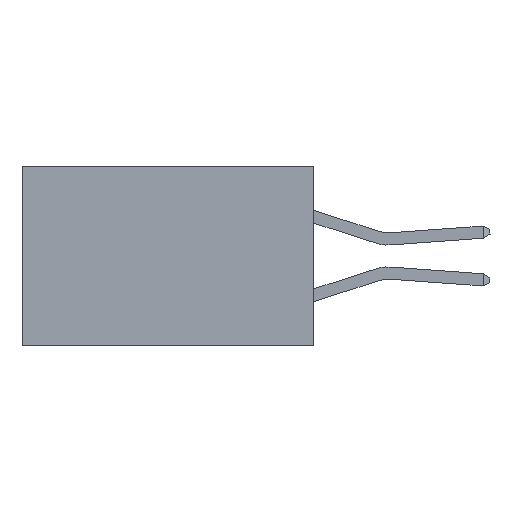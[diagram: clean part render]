
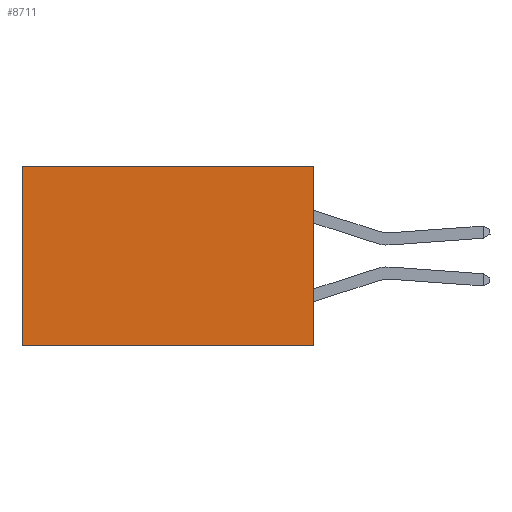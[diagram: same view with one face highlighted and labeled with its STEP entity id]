
A CAD part, left-side view. The second image highlights one B-rep face of the part: STEP entity #8711.
In plain terms, the highlighted planar face has unit normal (-1, 0, 0).
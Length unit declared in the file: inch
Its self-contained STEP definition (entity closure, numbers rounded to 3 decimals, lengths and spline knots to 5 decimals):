
#240 = LINE ( 'NONE', #2811, #2835 ) ;
#1067 = DIRECTION ( 'NONE',  ( 1., 0., 0. ) ) ;
#1459 = LINE ( 'NONE', #3209, #2245 ) ;
#2013 = CARTESIAN_POINT ( 'NONE',  ( 0.2875, 0., 0. ) ) ;
#2209 = CARTESIAN_POINT ( 'NONE',  ( 0.2875, 0., -0.37 ) ) ;
#2245 = VECTOR ( 'NONE', #2960, 39.37008 ) ;
#2811 = CARTESIAN_POINT ( 'NONE',  ( 0.2875, 0., -0.37 ) ) ;
#2835 = VECTOR ( 'NONE', #8566, 39.37008 ) ;
#2927 = LINE ( 'NONE', #10549, #6907 ) ;
#2960 = DIRECTION ( 'NONE',  ( 0., 1., 0. ) ) ;
#3209 = CARTESIAN_POINT ( 'NONE',  ( 0.2875, 0., 0. ) ) ;
#3832 = VERTEX_POINT ( 'NONE', #8491 ) ;
#3949 = EDGE_CURVE ( 'NONE', #9063, #3832, #240, .T. ) ;
#4190 = EDGE_CURVE ( 'NONE', #6216, #9063, #6421, .T. ) ;
#4245 = VECTOR ( 'NONE', #7698, 39.37008 ) ;
#4391 = EDGE_LOOP ( 'NONE', ( #4953, #5230, #9896, #4965 ) ) ;
#4953 = ORIENTED_EDGE ( 'NONE', *, *, #6367, .T. ) ;
#4965 = ORIENTED_EDGE ( 'NONE', *, *, #8217, .T. ) ;
#5230 = ORIENTED_EDGE ( 'NONE', *, *, #3949, .F. ) ;
#6216 = VERTEX_POINT ( 'NONE', #10643 ) ;
#6278 = DIRECTION ( 'NONE',  ( 0., 0., -1. ) ) ;
#6367 = EDGE_CURVE ( 'NONE', #9427, #3832, #2927, .T. ) ;
#6421 = LINE ( 'NONE', #2013, #4245 ) ;
#6615 = CARTESIAN_POINT ( 'NONE',  ( 0.2875, 0.6, 0. ) ) ;
#6892 = DIRECTION ( 'NONE',  ( 0., 0., -1. ) ) ;
#6907 = VECTOR ( 'NONE', #6278, 39.37008 ) ;
#7232 = FACE_OUTER_BOUND ( 'NONE', #4391, .T. ) ;
#7698 = DIRECTION ( 'NONE',  ( 0., 0., -1. ) ) ;
#7753 = PLANE ( 'NONE',  #8982 ) ;
#8217 = EDGE_CURVE ( 'NONE', #6216, #9427, #1459, .T. ) ;
#8491 = CARTESIAN_POINT ( 'NONE',  ( 0.2875, 0.6, -0.37 ) ) ;
#8522 = CARTESIAN_POINT ( 'NONE',  ( 0.2875, 0., 0. ) ) ;
#8566 = DIRECTION ( 'NONE',  ( 0., 1., 0. ) ) ;
#8711 = ADVANCED_FACE ( 'NONE', ( #7232 ), #7753, .F. ) ;
#8982 = AXIS2_PLACEMENT_3D ( 'NONE', #8522, #1067, #6892 ) ;
#9063 = VERTEX_POINT ( 'NONE', #2209 ) ;
#9427 = VERTEX_POINT ( 'NONE', #6615 ) ;
#9896 = ORIENTED_EDGE ( 'NONE', *, *, #4190, .F. ) ;
#10549 = CARTESIAN_POINT ( 'NONE',  ( 0.2875, 0.6, 0. ) ) ;
#10643 = CARTESIAN_POINT ( 'NONE',  ( 0.2875, 0., 0. ) ) ;
